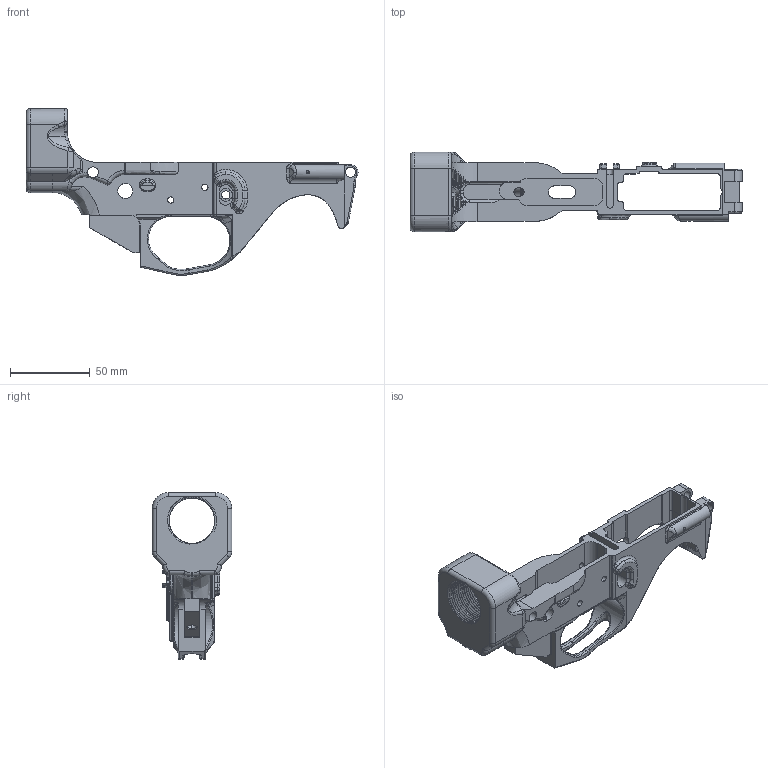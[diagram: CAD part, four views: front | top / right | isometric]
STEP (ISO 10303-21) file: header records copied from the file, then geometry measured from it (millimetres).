
FILE_DESCRIPTION (( 'STEP AP214' ), '1' );
FILE_NAME ('Hermes_Zero_V2.STEP', '2015-05-21T08:31:04', ( 'WarFairy' ), ( '' ), 'SwSTEP 2.0', 'SolidWorks 2015', '' );
FILE_SCHEMA (( 'AUTOMOTIVE_DESIGN' ));
Products named in the file (1): Hermes_Zero_V2
Bounding box: 208.83 x 50 x 104.96 mm (x, y, z)
Volume: 135191.5 mm3; surface area: 53721.5 mm2
Topology: 1 solids, 1 shells, 879 faces, 2424 edges, 1507 vertices
Faces by surface type: cylinder 371, bspline 285, plane 199, torus 13, sphere 6, cone 5
Entity records: 56410 total; most frequent: CARTESIAN_POINT 36891, ORIENTED_EDGE 4792, DIRECTION 3178, EDGE_CURVE 2396, VERTEX_POINT 1507, AXIS2_PLACEMENT_3D 1175, EDGE_LOOP 911, FACE_OUTER_BOUND 879
